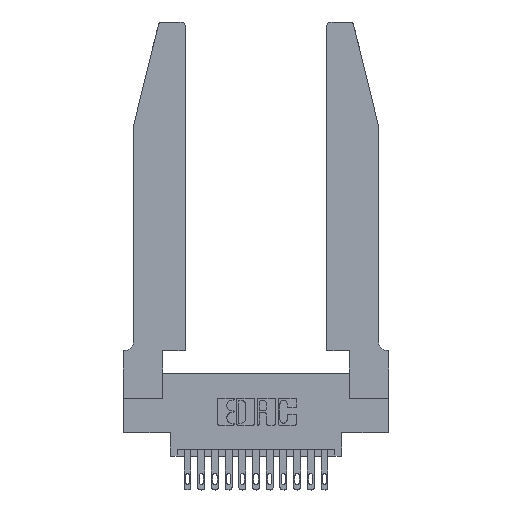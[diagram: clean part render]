
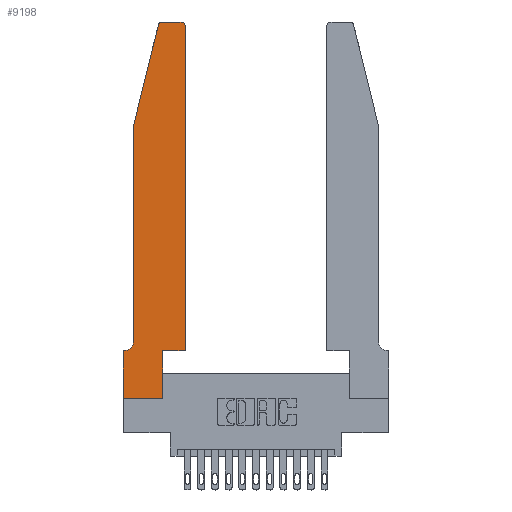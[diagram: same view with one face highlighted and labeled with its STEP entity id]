
A CAD part, top view. The second image highlights one B-rep face of the part: STEP entity #9198.
In plain terms, the highlighted planar face has unit normal (0, 0, 1).
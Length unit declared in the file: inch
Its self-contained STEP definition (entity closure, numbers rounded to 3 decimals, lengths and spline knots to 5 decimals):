
#70 = DIRECTION ( 'NONE',  ( -1., 0., 0. ) ) ;
#192 = DIRECTION ( 'NONE',  ( 1., 0., 0. ) ) ;
#253 = DIRECTION ( 'NONE',  ( 0., 0., 1. ) ) ;
#403 = EDGE_CURVE ( 'NONE', #13593, #6462, #7326, .T. ) ;
#1056 = VECTOR ( 'NONE', #13183, 39.37008 ) ;
#1723 = VECTOR ( 'NONE', #70, 39.37008 ) ;
#2063 = CARTESIAN_POINT ( 'NONE',  ( 0.0755, 0.42, 0.37 ) ) ;
#2256 = CIRCLE ( 'NONE', #17534, 0.03 ) ;
#2463 = VECTOR ( 'NONE', #9874, 39.37008 ) ;
#2491 = FACE_OUTER_BOUND ( 'NONE', #12542, .T. ) ;
#2522 = ORIENTED_EDGE ( 'NONE', *, *, #3325, .T. ) ;
#2651 = PLANE ( 'NONE',  #4009 ) ;
#2900 = DIRECTION ( 'NONE',  ( 0., 1., 0. ) ) ;
#3325 = EDGE_CURVE ( 'NONE', #15881, #15480, #16984, .T. ) ;
#3409 = DIRECTION ( 'NONE',  ( 0., 0., 1. ) ) ;
#3522 = CARTESIAN_POINT ( 'NONE',  ( 0.284, 2.72, 0.37 ) ) ;
#3939 = DIRECTION ( 'NONE',  ( 0., 0., -1. ) ) ;
#4009 = AXIS2_PLACEMENT_3D ( 'NONE', #12504, #253, #192 ) ;
#4155 = CARTESIAN_POINT ( 'NONE',  ( 0.4205, 2.75, 0.37 ) ) ;
#4199 = VERTEX_POINT ( 'NONE', #13713 ) ;
#4211 = LINE ( 'NONE', #7882, #10375 ) ;
#4342 = CARTESIAN_POINT ( 'NONE',  ( 0.4505, 2.72, 0.37 ) ) ;
#4442 = CARTESIAN_POINT ( 'NONE',  ( 0.2865, 0., 0.37 ) ) ;
#4714 = LINE ( 'NONE', #17123, #1723 ) ;
#4793 = VECTOR ( 'NONE', #5564, 39.37008 ) ;
#4960 = LINE ( 'NONE', #15576, #11787 ) ;
#5126 = EDGE_CURVE ( 'NONE', #15480, #5251, #8996, .T. ) ;
#5219 = CARTESIAN_POINT ( 'NONE',  ( 0., 0.35, 0.37 ) ) ;
#5251 = VERTEX_POINT ( 'NONE', #9240 ) ;
#5564 = DIRECTION ( 'NONE',  ( 1., 0., 0. ) ) ;
#5603 = EDGE_CURVE ( 'NONE', #10959, #15881, #9851, .T. ) ;
#5776 = VECTOR ( 'NONE', #15722, 39.37008 ) ;
#5801 = CARTESIAN_POINT ( 'NONE',  ( 0.4205, 2.72, 0.37 ) ) ;
#5822 = VECTOR ( 'NONE', #12384, 39.37008 ) ;
#5865 = ORIENTED_EDGE ( 'NONE', *, *, #15429, .T. ) ;
#5930 = ORIENTED_EDGE ( 'NONE', *, *, #15177, .T. ) ;
#6462 = VERTEX_POINT ( 'NONE', #10178 ) ;
#6502 = CARTESIAN_POINT ( 'NONE',  ( 0.0755, 2., 0.37 ) ) ;
#7093 = ORIENTED_EDGE ( 'NONE', *, *, #5126, .T. ) ;
#7123 = CARTESIAN_POINT ( 'NONE',  ( 0.0755, 0.35, 0.37 ) ) ;
#7326 = LINE ( 'NONE', #16541, #4793 ) ;
#7400 = CARTESIAN_POINT ( 'NONE',  ( 0.284, 2.75, 0.37 ) ) ;
#7882 = CARTESIAN_POINT ( 'NONE',  ( 0., 0., 0.37 ) ) ;
#7950 = DIRECTION ( 'NONE',  ( -1., 0., 0. ) ) ;
#8291 = AXIS2_PLACEMENT_3D ( 'NONE', #9318, #3939, #7950 ) ;
#8332 = VERTEX_POINT ( 'NONE', #10751 ) ;
#8996 = LINE ( 'NONE', #13925, #5822 ) ;
#9198 = ADVANCED_FACE ( 'NONE', ( #2491 ), #2651, .T. ) ;
#9240 = CARTESIAN_POINT ( 'NONE',  ( 0., 0., 0.37 ) ) ;
#9318 = CARTESIAN_POINT ( 'NONE',  ( 0.0055, 0.42, 0.37 ) ) ;
#9562 = EDGE_CURVE ( 'NONE', #8332, #4199, #12984, .T. ) ;
#9588 = DIRECTION ( 'NONE',  ( 0., 0., 1. ) ) ;
#9690 = CARTESIAN_POINT ( 'NONE',  ( 0.4505, 0.35, 0.37 ) ) ;
#9826 = LINE ( 'NONE', #11622, #5776 ) ;
#9851 = CIRCLE ( 'NONE', #8291, 0.07 ) ;
#9874 = DIRECTION ( 'NONE',  ( -1., 0., 0. ) ) ;
#10178 = CARTESIAN_POINT ( 'NONE',  ( 0.4505, 0.35, 0.37 ) ) ;
#10375 = VECTOR ( 'NONE', #17433, 39.37008 ) ;
#10380 = ORIENTED_EDGE ( 'NONE', *, *, #13563, .T. ) ;
#10703 = EDGE_CURVE ( 'NONE', #5251, #12172, #4211, .T. ) ;
#10751 = CARTESIAN_POINT ( 'NONE',  ( 0.25487, 2.72718, 0.37 ) ) ;
#10848 = VERTEX_POINT ( 'NONE', #4342 ) ;
#10959 = VERTEX_POINT ( 'NONE', #2063 ) ;
#11011 = ORIENTED_EDGE ( 'NONE', *, *, #11181, .T. ) ;
#11181 = EDGE_CURVE ( 'NONE', #10848, #14879, #15916, .T. ) ;
#11622 = CARTESIAN_POINT ( 'NONE',  ( 0.2865, 0.35, 0.37 ) ) ;
#11649 = LINE ( 'NONE', #9690, #16531 ) ;
#11787 = VECTOR ( 'NONE', #16760, 39.37008 ) ;
#11946 = EDGE_CURVE ( 'NONE', #6462, #10848, #11649, .T. ) ;
#12172 = VERTEX_POINT ( 'NONE', #4442 ) ;
#12362 = AXIS2_PLACEMENT_3D ( 'NONE', #5801, #9588, #15370 ) ;
#12384 = DIRECTION ( 'NONE',  ( 0., -1., 0. ) ) ;
#12504 = CARTESIAN_POINT ( 'NONE',  ( 0., 0.35, 0.37 ) ) ;
#12542 = EDGE_LOOP ( 'NONE', ( #5865, #13555, #14134, #10380, #17519, #2522, #7093, #12714, #5930, #17475, #12693, #11011 ) ) ;
#12693 = ORIENTED_EDGE ( 'NONE', *, *, #11946, .T. ) ;
#12714 = ORIENTED_EDGE ( 'NONE', *, *, #10703, .T. ) ;
#12984 = LINE ( 'NONE', #6502, #1056 ) ;
#13057 = DIRECTION ( 'NONE',  ( 1., 0., 0. ) ) ;
#13183 = DIRECTION ( 'NONE',  ( -0.239, -0.971, 0. ) ) ;
#13287 = CARTESIAN_POINT ( 'NONE',  ( 0.0055, 0.35, 0.37 ) ) ;
#13555 = ORIENTED_EDGE ( 'NONE', *, *, #16315, .T. ) ;
#13563 = EDGE_CURVE ( 'NONE', #4199, #10959, #4960, .T. ) ;
#13593 = VERTEX_POINT ( 'NONE', #16921 ) ;
#13713 = CARTESIAN_POINT ( 'NONE',  ( 0.0755, 2., 0.37 ) ) ;
#13925 = CARTESIAN_POINT ( 'NONE',  ( 0., 0., 0.37 ) ) ;
#14134 = ORIENTED_EDGE ( 'NONE', *, *, #9562, .T. ) ;
#14879 = VERTEX_POINT ( 'NONE', #4155 ) ;
#15177 = EDGE_CURVE ( 'NONE', #12172, #13593, #9826, .T. ) ;
#15370 = DIRECTION ( 'NONE',  ( 1., 0., 0. ) ) ;
#15429 = EDGE_CURVE ( 'NONE', #14879, #17367, #4714, .T. ) ;
#15480 = VERTEX_POINT ( 'NONE', #5219 ) ;
#15576 = CARTESIAN_POINT ( 'NONE',  ( 0.0755, 2., 0.37 ) ) ;
#15722 = DIRECTION ( 'NONE',  ( 0., 1., 0. ) ) ;
#15881 = VERTEX_POINT ( 'NONE', #13287 ) ;
#15916 = CIRCLE ( 'NONE', #12362, 0.03 ) ;
#16315 = EDGE_CURVE ( 'NONE', #17367, #8332, #2256, .T. ) ;
#16531 = VECTOR ( 'NONE', #2900, 39.37008 ) ;
#16541 = CARTESIAN_POINT ( 'NONE',  ( 0.4505, 0.35, 0.37 ) ) ;
#16760 = DIRECTION ( 'NONE',  ( 0., -1., 0. ) ) ;
#16921 = CARTESIAN_POINT ( 'NONE',  ( 0.2865, 0.35, 0.37 ) ) ;
#16984 = LINE ( 'NONE', #7123, #2463 ) ;
#17123 = CARTESIAN_POINT ( 'NONE',  ( 0.2605, 2.75, 0.37 ) ) ;
#17367 = VERTEX_POINT ( 'NONE', #7400 ) ;
#17433 = DIRECTION ( 'NONE',  ( 1., 0., 0. ) ) ;
#17475 = ORIENTED_EDGE ( 'NONE', *, *, #403, .T. ) ;
#17519 = ORIENTED_EDGE ( 'NONE', *, *, #5603, .T. ) ;
#17534 = AXIS2_PLACEMENT_3D ( 'NONE', #3522, #3409, #13057 ) ;
